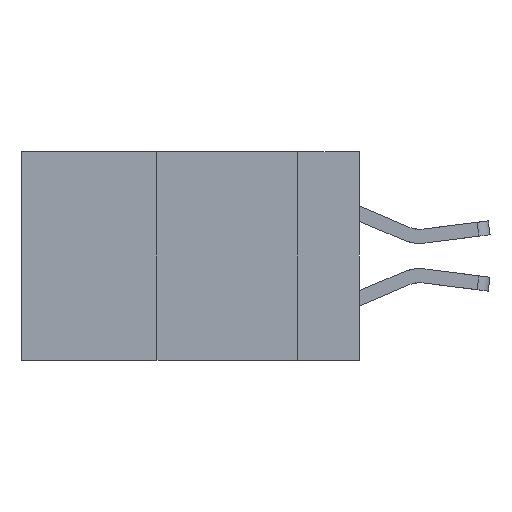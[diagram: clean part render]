
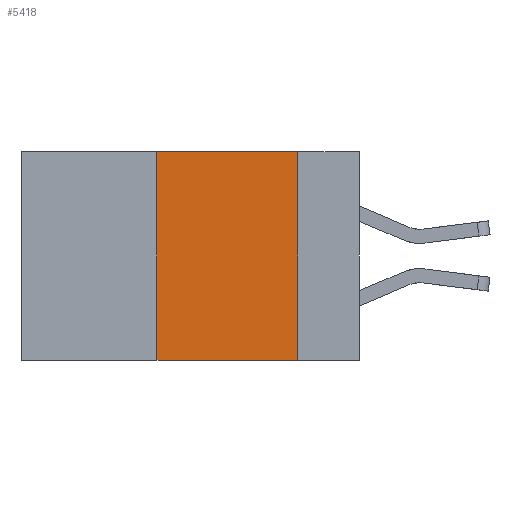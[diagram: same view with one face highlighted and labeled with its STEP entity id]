
A CAD part, left-side view. The second image highlights one B-rep face of the part: STEP entity #5418.
In plain terms, the highlighted planar face has unit normal (-1, 0, 0).
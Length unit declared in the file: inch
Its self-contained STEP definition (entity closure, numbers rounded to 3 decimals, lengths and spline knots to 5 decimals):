
#85 = ORIENTED_EDGE ( 'NONE', *, *, #12741, .F. ) ;
#800 = FACE_OUTER_BOUND ( 'NONE', #9874, .T. ) ;
#878 = AXIS2_PLACEMENT_3D ( 'NONE', #3734, #1558, #7640 ) ;
#1175 = VERTEX_POINT ( 'NONE', #13023 ) ;
#1207 = EDGE_CURVE ( 'NONE', #6813, #5911, #10432, .T. ) ;
#1245 = CARTESIAN_POINT ( 'NONE',  ( 0., 0.6, 0. ) ) ;
#1359 = PLANE ( 'NONE',  #878 ) ;
#1558 = DIRECTION ( 'NONE',  ( 1., 0., 0. ) ) ;
#1616 = ORIENTED_EDGE ( 'NONE', *, *, #1207, .F. ) ;
#1934 = ORIENTED_EDGE ( 'NONE', *, *, #5545, .T. ) ;
#2030 = DIRECTION ( 'NONE',  ( 0., 0., -1. ) ) ;
#3315 = VERTEX_POINT ( 'NONE', #10874 ) ;
#3734 = CARTESIAN_POINT ( 'NONE',  ( 0., 0.6, 0. ) ) ;
#4221 = CARTESIAN_POINT ( 'NONE',  ( 0., 0.6, -0.37 ) ) ;
#4835 = VECTOR ( 'NONE', #7307, 39.37008 ) ;
#5044 = CARTESIAN_POINT ( 'NONE',  ( 0., 0.11, 0. ) ) ;
#5295 = CARTESIAN_POINT ( 'NONE',  ( 0., 0.36, -0.37 ) ) ;
#5418 = ADVANCED_FACE ( 'NONE', ( #800 ), #1359, .F. ) ;
#5545 = EDGE_CURVE ( 'NONE', #6813, #3315, #7243, .T. ) ;
#5720 = DIRECTION ( 'NONE',  ( 0., 0., 1. ) ) ;
#5739 = DIRECTION ( 'NONE',  ( 0., -1., 0. ) ) ;
#5853 = CARTESIAN_POINT ( 'NONE',  ( 0., 0.36, 0. ) ) ;
#5911 = VERTEX_POINT ( 'NONE', #9689 ) ;
#6813 = VERTEX_POINT ( 'NONE', #5295 ) ;
#7243 = LINE ( 'NONE', #4221, #4835 ) ;
#7307 = DIRECTION ( 'NONE',  ( 0., -1., 0. ) ) ;
#7640 = DIRECTION ( 'NONE',  ( 0., 0., -1. ) ) ;
#7680 = VECTOR ( 'NONE', #5720, 39.37008 ) ;
#8251 = LINE ( 'NONE', #5044, #8900 ) ;
#8900 = VECTOR ( 'NONE', #2030, 39.37008 ) ;
#8929 = LINE ( 'NONE', #1245, #11333 ) ;
#9689 = CARTESIAN_POINT ( 'NONE',  ( 0., 0.36, 0. ) ) ;
#9874 = EDGE_LOOP ( 'NONE', ( #85, #12022, #1616, #1934 ) ) ;
#10432 = LINE ( 'NONE', #5853, #7680 ) ;
#10874 = CARTESIAN_POINT ( 'NONE',  ( 0., 0.11, -0.37 ) ) ;
#11333 = VECTOR ( 'NONE', #5739, 39.37008 ) ;
#11876 = EDGE_CURVE ( 'NONE', #5911, #1175, #8929, .T. ) ;
#12022 = ORIENTED_EDGE ( 'NONE', *, *, #11876, .F. ) ;
#12741 = EDGE_CURVE ( 'NONE', #1175, #3315, #8251, .T. ) ;
#13023 = CARTESIAN_POINT ( 'NONE',  ( 0., 0.11, 0. ) ) ;
